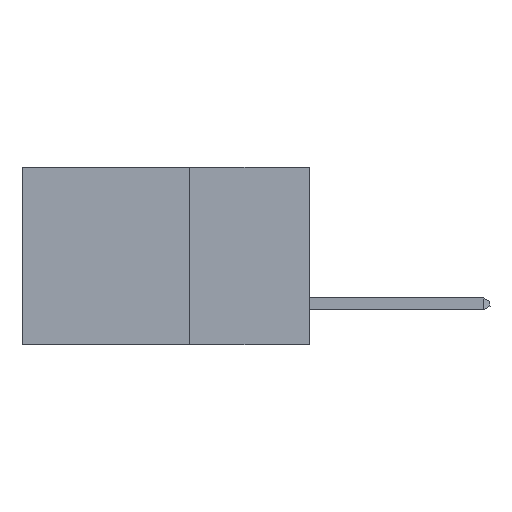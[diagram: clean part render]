
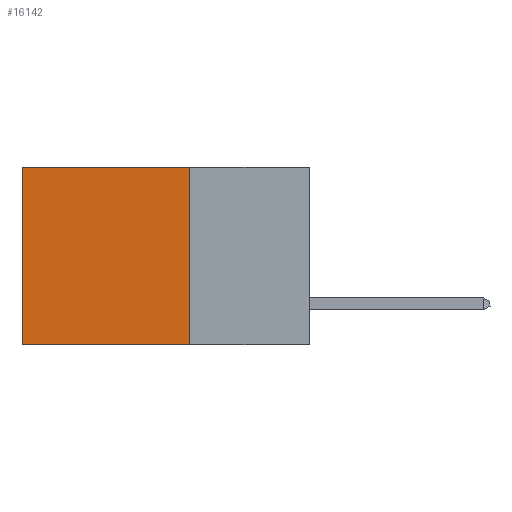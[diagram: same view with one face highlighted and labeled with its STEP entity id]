
A CAD part, left-side view. The second image highlights one B-rep face of the part: STEP entity #16142.
In plain terms, the highlighted planar face has unit normal (-1, 0, 0).
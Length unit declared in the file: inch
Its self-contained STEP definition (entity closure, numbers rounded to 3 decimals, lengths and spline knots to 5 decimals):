
#227 = FACE_OUTER_BOUND ( 'NONE', #25693, .T. ) ;
#2322 = DIRECTION ( 'NONE',  ( 0., 1., 0. ) ) ;
#2553 = CARTESIAN_POINT ( 'NONE',  ( 0.2875, 0.6, -0.37 ) ) ;
#3309 = VECTOR ( 'NONE', #4633, 39.37008 ) ;
#4507 = LINE ( 'NONE', #29569, #9995 ) ;
#4633 = DIRECTION ( 'NONE',  ( 0., 1., 0. ) ) ;
#6574 = PLANE ( 'NONE',  #23047 ) ;
#8619 = CARTESIAN_POINT ( 'NONE',  ( 0.2875, 0.6, 0. ) ) ;
#9995 = VECTOR ( 'NONE', #13816, 39.37008 ) ;
#10964 = DIRECTION ( 'NONE',  ( 0., 0., -1. ) ) ;
#11454 = VERTEX_POINT ( 'NONE', #2553 ) ;
#11928 = LINE ( 'NONE', #8619, #16544 ) ;
#12386 = VERTEX_POINT ( 'NONE', #26420 ) ;
#13252 = ORIENTED_EDGE ( 'NONE', *, *, #29185, .F. ) ;
#13623 = DIRECTION ( 'NONE',  ( 1., 0., 0. ) ) ;
#13816 = DIRECTION ( 'NONE',  ( 0., 0., -1. ) ) ;
#14481 = ORIENTED_EDGE ( 'NONE', *, *, #22273, .T. ) ;
#15679 = LINE ( 'NONE', #16279, #3309 ) ;
#15716 = VECTOR ( 'NONE', #2322, 39.37008 ) ;
#16142 = ADVANCED_FACE ( 'NONE', ( #227 ), #6574, .F. ) ;
#16253 = ORIENTED_EDGE ( 'NONE', *, *, #24786, .T. ) ;
#16279 = CARTESIAN_POINT ( 'NONE',  ( 0.2875, 0.25, 0. ) ) ;
#16544 = VECTOR ( 'NONE', #10964, 39.37008 ) ;
#21708 = CARTESIAN_POINT ( 'NONE',  ( 0.2875, 0.6, 0. ) ) ;
#22273 = EDGE_CURVE ( 'NONE', #24412, #11454, #11928, .T. ) ;
#22571 = VERTEX_POINT ( 'NONE', #23319 ) ;
#22909 = CARTESIAN_POINT ( 'NONE',  ( 0.2875, 0.25, -0.37 ) ) ;
#23047 = AXIS2_PLACEMENT_3D ( 'NONE', #27101, #13623, #29382 ) ;
#23319 = CARTESIAN_POINT ( 'NONE',  ( 0.2875, 0.25, -0.37 ) ) ;
#23389 = ORIENTED_EDGE ( 'NONE', *, *, #28511, .F. ) ;
#24412 = VERTEX_POINT ( 'NONE', #21708 ) ;
#24786 = EDGE_CURVE ( 'NONE', #12386, #24412, #15679, .T. ) ;
#25693 = EDGE_LOOP ( 'NONE', ( #14481, #13252, #23389, #16253 ) ) ;
#26420 = CARTESIAN_POINT ( 'NONE',  ( 0.2875, 0.25, 0. ) ) ;
#27101 = CARTESIAN_POINT ( 'NONE',  ( 0.2875, 0.25, 0. ) ) ;
#27695 = LINE ( 'NONE', #22909, #15716 ) ;
#28511 = EDGE_CURVE ( 'NONE', #12386, #22571, #4507, .T. ) ;
#29185 = EDGE_CURVE ( 'NONE', #22571, #11454, #27695, .T. ) ;
#29382 = DIRECTION ( 'NONE',  ( 0., 0., -1. ) ) ;
#29569 = CARTESIAN_POINT ( 'NONE',  ( 0.2875, 0.25, 0. ) ) ;
